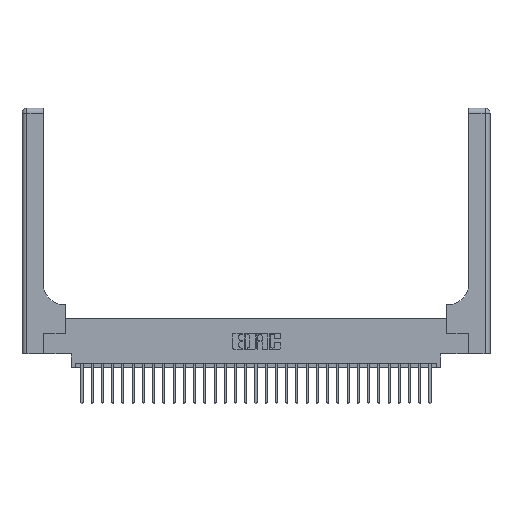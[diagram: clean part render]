
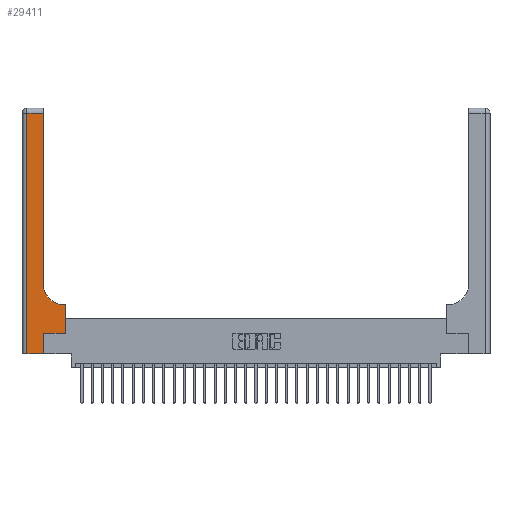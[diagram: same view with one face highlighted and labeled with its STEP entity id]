
A CAD part, top view. The second image highlights one B-rep face of the part: STEP entity #29411.
In plain terms, the highlighted planar face has unit normal (0, 0, 1).
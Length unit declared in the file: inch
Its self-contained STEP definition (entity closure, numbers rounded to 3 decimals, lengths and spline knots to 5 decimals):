
#261 = VERTEX_POINT ( 'NONE', #27706 ) ;
#640 = ORIENTED_EDGE ( 'NONE', *, *, #12458, .T. ) ;
#641 = DIRECTION ( 'NONE',  ( 0., 1., 0. ) ) ;
#692 = ORIENTED_EDGE ( 'NONE', *, *, #25626, .T. ) ;
#823 = CARTESIAN_POINT ( 'NONE',  ( 0.06, 2.94, 0.37 ) ) ;
#1195 = DIRECTION ( 'NONE',  ( 0., -1., 0. ) ) ;
#1341 = LINE ( 'NONE', #5990, #7998 ) ;
#1993 = VECTOR ( 'NONE', #641, 39.37008 ) ;
#2025 = CARTESIAN_POINT ( 'NONE',  ( 0.265, 0., 0.37 ) ) ;
#2123 = CIRCLE ( 'NONE', #4522, 0.25 ) ;
#2647 = DIRECTION ( 'NONE',  ( 1., 0., 0. ) ) ;
#3037 = VERTEX_POINT ( 'NONE', #2025 ) ;
#3885 = VERTEX_POINT ( 'NONE', #4353 ) ;
#4295 = EDGE_CURVE ( 'NONE', #3037, #3885, #17216, .T. ) ;
#4353 = CARTESIAN_POINT ( 'NONE',  ( 0.265, 0.25, 0.37 ) ) ;
#4522 = AXIS2_PLACEMENT_3D ( 'NONE', #6214, #8162, #24320 ) ;
#5017 = VERTEX_POINT ( 'NONE', #10233 ) ;
#5695 = CARTESIAN_POINT ( 'NONE',  ( 0.06, 3., 0.37 ) ) ;
#5990 = CARTESIAN_POINT ( 'NONE',  ( 0., 2.94, 0.37 ) ) ;
#6214 = CARTESIAN_POINT ( 'NONE',  ( 0.51, 0.85, 0.37 ) ) ;
#6526 = VERTEX_POINT ( 'NONE', #21375 ) ;
#6654 = CARTESIAN_POINT ( 'NONE',  ( 0.265, 0.25, 0.37 ) ) ;
#7007 = LINE ( 'NONE', #25120, #20391 ) ;
#7998 = VECTOR ( 'NONE', #15123, 39.37008 ) ;
#8081 = FACE_OUTER_BOUND ( 'NONE', #14337, .T. ) ;
#8162 = DIRECTION ( 'NONE',  ( 0., 0., -1. ) ) ;
#8183 = ORIENTED_EDGE ( 'NONE', *, *, #4295, .T. ) ;
#8711 = EDGE_CURVE ( 'NONE', #3885, #17864, #9037, .T. ) ;
#9037 = LINE ( 'NONE', #6654, #19304 ) ;
#9457 = AXIS2_PLACEMENT_3D ( 'NONE', #25881, #14514, #23644 ) ;
#10233 = CARTESIAN_POINT ( 'NONE',  ( 0.51, 0.6, 0.37 ) ) ;
#10912 = CARTESIAN_POINT ( 'NONE',  ( 0.528, 0.25, 0.37 ) ) ;
#12300 = VERTEX_POINT ( 'NONE', #823 ) ;
#12331 = LINE ( 'NONE', #19084, #1993 ) ;
#12458 = EDGE_CURVE ( 'NONE', #5017, #6526, #2123, .T. ) ;
#12860 = LINE ( 'NONE', #10912, #26101 ) ;
#13286 = VERTEX_POINT ( 'NONE', #20324 ) ;
#13482 = DIRECTION ( 'NONE',  ( -1., 0., 0. ) ) ;
#13739 = ORIENTED_EDGE ( 'NONE', *, *, #22730, .T. ) ;
#14072 = EDGE_CURVE ( 'NONE', #6526, #28056, #12331, .T. ) ;
#14337 = EDGE_LOOP ( 'NONE', ( #22475, #692, #19970, #18771, #8183, #18012, #13739, #22168, #640 ) ) ;
#14514 = DIRECTION ( 'NONE',  ( 0., 0., -1. ) ) ;
#15123 = DIRECTION ( 'NONE',  ( -1., 0., 0. ) ) ;
#15592 = LINE ( 'NONE', #24413, #15909 ) ;
#15776 = DIRECTION ( 'NONE',  ( 1., 0., 0. ) ) ;
#15909 = VECTOR ( 'NONE', #13482, 39.37008 ) ;
#17079 = LINE ( 'NONE', #5695, #25365 ) ;
#17216 = LINE ( 'NONE', #19627, #19265 ) ;
#17286 = EDGE_CURVE ( 'NONE', #261, #5017, #15592, .T. ) ;
#17864 = VERTEX_POINT ( 'NONE', #21678 ) ;
#18012 = ORIENTED_EDGE ( 'NONE', *, *, #8711, .T. ) ;
#18771 = ORIENTED_EDGE ( 'NONE', *, *, #22834, .T. ) ;
#19084 = CARTESIAN_POINT ( 'NONE',  ( 0.26, 3., 0.37 ) ) ;
#19265 = VECTOR ( 'NONE', #26333, 39.37008 ) ;
#19304 = VECTOR ( 'NONE', #15776, 39.37008 ) ;
#19354 = EDGE_CURVE ( 'NONE', #12300, #13286, #17079, .T. ) ;
#19627 = CARTESIAN_POINT ( 'NONE',  ( 0.265, 0., 0.37 ) ) ;
#19970 = ORIENTED_EDGE ( 'NONE', *, *, #19354, .T. ) ;
#20324 = CARTESIAN_POINT ( 'NONE',  ( 0.06, 0., 0.37 ) ) ;
#20391 = VECTOR ( 'NONE', #2647, 39.37008 ) ;
#21375 = CARTESIAN_POINT ( 'NONE',  ( 0.26, 0.85, 0.37 ) ) ;
#21678 = CARTESIAN_POINT ( 'NONE',  ( 0.528, 0.25, 0.37 ) ) ;
#21994 = DIRECTION ( 'NONE',  ( 0., 1., 0. ) ) ;
#22168 = ORIENTED_EDGE ( 'NONE', *, *, #17286, .T. ) ;
#22475 = ORIENTED_EDGE ( 'NONE', *, *, #14072, .T. ) ;
#22730 = EDGE_CURVE ( 'NONE', #17864, #261, #12860, .T. ) ;
#22834 = EDGE_CURVE ( 'NONE', #13286, #3037, #7007, .T. ) ;
#23644 = DIRECTION ( 'NONE',  ( -1., 0., 0. ) ) ;
#24320 = DIRECTION ( 'NONE',  ( 1., 0., 0. ) ) ;
#24413 = CARTESIAN_POINT ( 'NONE',  ( 0.26, 0.6, 0.37 ) ) ;
#25120 = CARTESIAN_POINT ( 'NONE',  ( 0., 0., 0.37 ) ) ;
#25365 = VECTOR ( 'NONE', #1195, 39.37008 ) ;
#25626 = EDGE_CURVE ( 'NONE', #28056, #12300, #1341, .T. ) ;
#25881 = CARTESIAN_POINT ( 'NONE',  ( 0., 3., 0.37 ) ) ;
#26101 = VECTOR ( 'NONE', #21994, 39.37008 ) ;
#26333 = DIRECTION ( 'NONE',  ( 0., 1., 0. ) ) ;
#27706 = CARTESIAN_POINT ( 'NONE',  ( 0.528, 0.6, 0.37 ) ) ;
#28056 = VERTEX_POINT ( 'NONE', #28821 ) ;
#28134 = PLANE ( 'NONE',  #9457 ) ;
#28821 = CARTESIAN_POINT ( 'NONE',  ( 0.26, 2.94, 0.37 ) ) ;
#29411 = ADVANCED_FACE ( 'NONE', ( #8081 ), #28134, .F. ) ;
